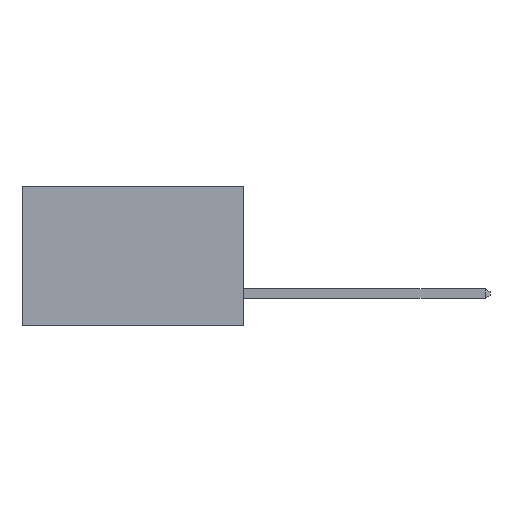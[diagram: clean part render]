
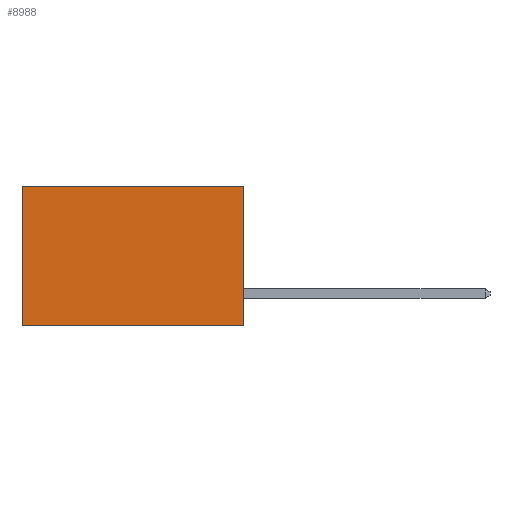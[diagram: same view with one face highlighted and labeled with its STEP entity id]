
A CAD part, left-side view. The second image highlights one B-rep face of the part: STEP entity #8988.
In plain terms, the highlighted planar face has unit normal (-1, 0, 0).
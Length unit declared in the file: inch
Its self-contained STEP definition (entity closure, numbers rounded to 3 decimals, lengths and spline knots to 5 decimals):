
#119 = EDGE_LOOP ( 'NONE', ( #352, #459, #541, #685 ) ) ;
#250 = CARTESIAN_POINT ( 'NONE',  ( 0.277, 0., -0.37 ) ) ;
#280 = DIRECTION ( 'NONE',  ( 0., 0., -1. ) ) ;
#352 = ORIENTED_EDGE ( 'NONE', *, *, #9631, .T. ) ;
#459 = ORIENTED_EDGE ( 'NONE', *, *, #3377, .F. ) ;
#541 = ORIENTED_EDGE ( 'NONE', *, *, #7261, .F. ) ;
#685 = ORIENTED_EDGE ( 'NONE', *, *, #1263, .T. ) ;
#1163 = CARTESIAN_POINT ( 'NONE',  ( 0.277, 0.59, -0.37 ) ) ;
#1181 = DIRECTION ( 'NONE',  ( 1., 0., 0. ) ) ;
#1263 = EDGE_CURVE ( 'NONE', #3674, #7538, #1402, .T. ) ;
#1360 = CARTESIAN_POINT ( 'NONE',  ( 0.277, 0.59, -0.37 ) ) ;
#1402 = LINE ( 'NONE', #7911, #3689 ) ;
#2710 = VERTEX_POINT ( 'NONE', #8544 ) ;
#3016 = CARTESIAN_POINT ( 'NONE',  ( 0.277, 0.59, 0. ) ) ;
#3233 = AXIS2_PLACEMENT_3D ( 'NONE', #250, #1181, #6881 ) ;
#3377 = EDGE_CURVE ( 'NONE', #2710, #4126, #7883, .T. ) ;
#3428 = VECTOR ( 'NONE', #6667, 39.37008 ) ;
#3562 = CARTESIAN_POINT ( 'NONE',  ( 0.277, 0., 0. ) ) ;
#3674 = VERTEX_POINT ( 'NONE', #3562 ) ;
#3689 = VECTOR ( 'NONE', #6749, 39.37008 ) ;
#3778 = LINE ( 'NONE', #1163, #7660 ) ;
#4126 = VERTEX_POINT ( 'NONE', #1360 ) ;
#4888 = DIRECTION ( 'NONE',  ( 0., 1., 0. ) ) ;
#5356 = PLANE ( 'NONE',  #3233 ) ;
#5560 = LINE ( 'NONE', #5906, #3428 ) ;
#5668 = CARTESIAN_POINT ( 'NONE',  ( 0.277, 0., -0.37 ) ) ;
#5860 = VECTOR ( 'NONE', #4888, 39.37008 ) ;
#5906 = CARTESIAN_POINT ( 'NONE',  ( 0.277, 0., -0.37 ) ) ;
#6667 = DIRECTION ( 'NONE',  ( 0., 0., -1. ) ) ;
#6749 = DIRECTION ( 'NONE',  ( 0., 1., 0. ) ) ;
#6881 = DIRECTION ( 'NONE',  ( 0., 0., -1. ) ) ;
#7261 = EDGE_CURVE ( 'NONE', #3674, #2710, #5560, .T. ) ;
#7538 = VERTEX_POINT ( 'NONE', #3016 ) ;
#7660 = VECTOR ( 'NONE', #280, 39.37008 ) ;
#7883 = LINE ( 'NONE', #5668, #5860 ) ;
#7911 = CARTESIAN_POINT ( 'NONE',  ( 0.277, 0., 0. ) ) ;
#8233 = FACE_OUTER_BOUND ( 'NONE', #119, .T. ) ;
#8544 = CARTESIAN_POINT ( 'NONE',  ( 0.277, 0., -0.37 ) ) ;
#8988 = ADVANCED_FACE ( 'NONE', ( #8233 ), #5356, .F. ) ;
#9631 = EDGE_CURVE ( 'NONE', #7538, #4126, #3778, .T. ) ;
